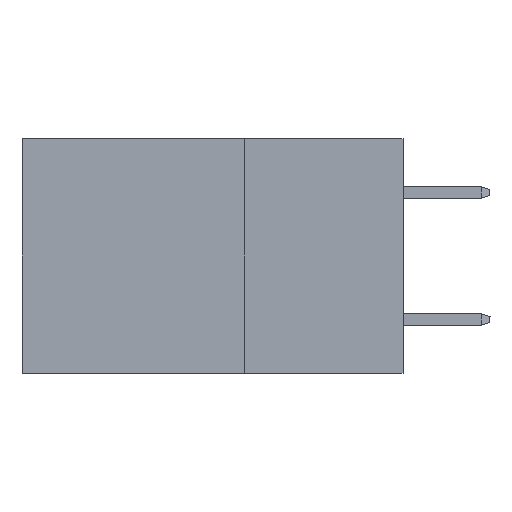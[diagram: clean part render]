
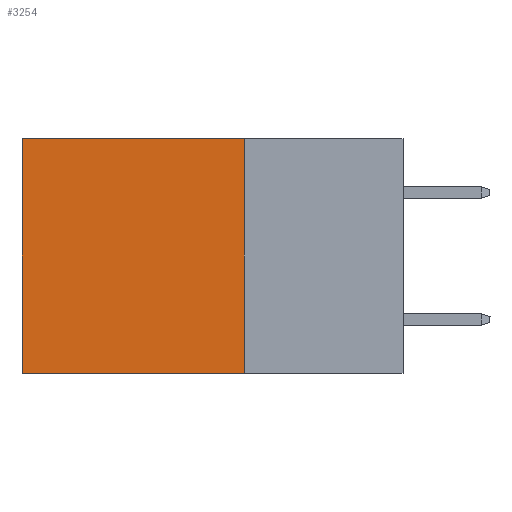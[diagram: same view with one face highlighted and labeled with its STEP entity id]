
A CAD part, left-side view. The second image highlights one B-rep face of the part: STEP entity #3254.
In plain terms, the highlighted planar face has unit normal (-1, 0, 0).
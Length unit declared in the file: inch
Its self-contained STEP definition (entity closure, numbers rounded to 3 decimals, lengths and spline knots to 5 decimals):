
#220 = CARTESIAN_POINT ( 'NONE',  ( 0.2875, 0.25, 0. ) ) ;
#1058 = VECTOR ( 'NONE', #23717, 39.37008 ) ;
#3254 = ADVANCED_FACE ( 'NONE', ( #14512 ), #18756, .F. ) ;
#3552 = DIRECTION ( 'NONE',  ( 1., 0., 0. ) ) ;
#3647 = ORIENTED_EDGE ( 'NONE', *, *, #9561, .T. ) ;
#4171 = VERTEX_POINT ( 'NONE', #220 ) ;
#4302 = CARTESIAN_POINT ( 'NONE',  ( 0.2875, 0.25, 0. ) ) ;
#4350 = CARTESIAN_POINT ( 'NONE',  ( 0.2875, 0.6, -0.37 ) ) ;
#4650 = VERTEX_POINT ( 'NONE', #4350 ) ;
#6192 = AXIS2_PLACEMENT_3D ( 'NONE', #10268, #3552, #16561 ) ;
#7542 = VECTOR ( 'NONE', #17630, 39.37008 ) ;
#8884 = CARTESIAN_POINT ( 'NONE',  ( 0.2875, 0.6, 0. ) ) ;
#9264 = ORIENTED_EDGE ( 'NONE', *, *, #10835, .F. ) ;
#9561 = EDGE_CURVE ( 'NONE', #24039, #4650, #21250, .T. ) ;
#10268 = CARTESIAN_POINT ( 'NONE',  ( 0.2875, 0.25, 0. ) ) ;
#10479 = VECTOR ( 'NONE', #12529, 39.37008 ) ;
#10835 = EDGE_CURVE ( 'NONE', #22200, #4650, #12389, .T. ) ;
#12389 = LINE ( 'NONE', #25242, #18198 ) ;
#12529 = DIRECTION ( 'NONE',  ( 0., 0., -1. ) ) ;
#12829 = EDGE_LOOP ( 'NONE', ( #3647, #9264, #22953, #14160 ) ) ;
#13664 = LINE ( 'NONE', #17774, #7542 ) ;
#14160 = ORIENTED_EDGE ( 'NONE', *, *, #26023, .T. ) ;
#14512 = FACE_OUTER_BOUND ( 'NONE', #12829, .T. ) ;
#16561 = DIRECTION ( 'NONE',  ( 0., 0., -1. ) ) ;
#17630 = DIRECTION ( 'NONE',  ( 0., 1., 0. ) ) ;
#17774 = CARTESIAN_POINT ( 'NONE',  ( 0.2875, 0.25, 0. ) ) ;
#18198 = VECTOR ( 'NONE', #25115, 39.37008 ) ;
#18756 = PLANE ( 'NONE',  #6192 ) ;
#21250 = LINE ( 'NONE', #25774, #1058 ) ;
#22200 = VERTEX_POINT ( 'NONE', #25885 ) ;
#22935 = EDGE_CURVE ( 'NONE', #4171, #22200, #27043, .T. ) ;
#22953 = ORIENTED_EDGE ( 'NONE', *, *, #22935, .F. ) ;
#23717 = DIRECTION ( 'NONE',  ( 0., 0., -1. ) ) ;
#24039 = VERTEX_POINT ( 'NONE', #8884 ) ;
#25115 = DIRECTION ( 'NONE',  ( 0., 1., 0. ) ) ;
#25242 = CARTESIAN_POINT ( 'NONE',  ( 0.2875, 0.25, -0.37 ) ) ;
#25774 = CARTESIAN_POINT ( 'NONE',  ( 0.2875, 0.6, 0. ) ) ;
#25885 = CARTESIAN_POINT ( 'NONE',  ( 0.2875, 0.25, -0.37 ) ) ;
#26023 = EDGE_CURVE ( 'NONE', #4171, #24039, #13664, .T. ) ;
#27043 = LINE ( 'NONE', #4302, #10479 ) ;
